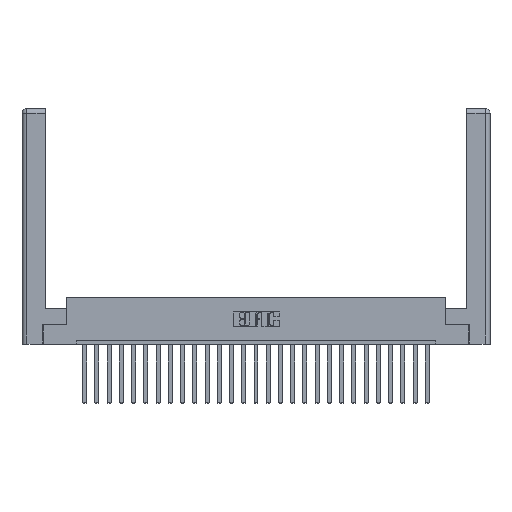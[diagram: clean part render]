
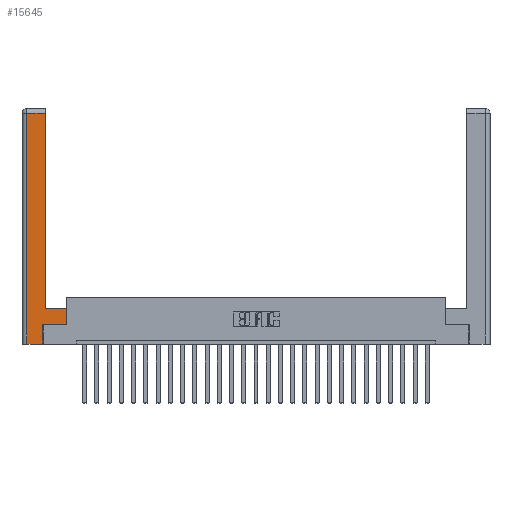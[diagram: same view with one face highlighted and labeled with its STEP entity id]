
A CAD part, top view. The second image highlights one B-rep face of the part: STEP entity #15645.
In plain terms, the highlighted planar face has unit normal (0, 0, 1).
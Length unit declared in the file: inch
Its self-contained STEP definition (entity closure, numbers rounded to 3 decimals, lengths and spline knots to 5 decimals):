
#399 = EDGE_CURVE ( 'NONE', #15824, #610, #18422, .T. ) ;
#425 = VERTEX_POINT ( 'NONE', #15621 ) ;
#495 = VECTOR ( 'NONE', #24600, 39.37008 ) ;
#610 = VERTEX_POINT ( 'NONE', #16352 ) ;
#700 = ORIENTED_EDGE ( 'NONE', *, *, #6892, .T. ) ;
#1013 = VECTOR ( 'NONE', #6196, 39.37008 ) ;
#1184 = VERTEX_POINT ( 'NONE', #17019 ) ;
#1859 = EDGE_CURVE ( 'NONE', #1184, #15824, #9740, .T. ) ;
#1968 = VERTEX_POINT ( 'NONE', #3947 ) ;
#2933 = ORIENTED_EDGE ( 'NONE', *, *, #16613, .T. ) ;
#3351 = ORIENTED_EDGE ( 'NONE', *, *, #1859, .T. ) ;
#3456 = CARTESIAN_POINT ( 'NONE',  ( 0., 0., 0. ) ) ;
#3850 = DIRECTION ( 'NONE',  ( 0., 1., 0. ) ) ;
#3947 = CARTESIAN_POINT ( 'NONE',  ( 0.295, 0.45, 0. ) ) ;
#5816 = LINE ( 'NONE', #20457, #495 ) ;
#6196 = DIRECTION ( 'NONE',  ( 0., -1., 0. ) ) ;
#6818 = DIRECTION ( 'NONE',  ( 1., 0., 0. ) ) ;
#6892 = EDGE_CURVE ( 'NONE', #16676, #21559, #5816, .T. ) ;
#8018 = DIRECTION ( 'NONE',  ( 1., 0., 0. ) ) ;
#8739 = VECTOR ( 'NONE', #8018, 39.37008 ) ;
#9120 = EDGE_CURVE ( 'NONE', #1968, #16676, #12401, .T. ) ;
#9267 = ORIENTED_EDGE ( 'NONE', *, *, #9120, .T. ) ;
#9740 = LINE ( 'NONE', #20321, #14400 ) ;
#9789 = VECTOR ( 'NONE', #11743, 39.37008 ) ;
#9829 = CARTESIAN_POINT ( 'NONE',  ( 0.565, 0.45, 0. ) ) ;
#10383 = EDGE_LOOP ( 'NONE', ( #9267, #700, #13866, #15862, #23009, #3351, #13496, #2933 ) ) ;
#10463 = VECTOR ( 'NONE', #19411, 39.37008 ) ;
#11362 = DIRECTION ( 'NONE',  ( -1., 0., 0. ) ) ;
#11571 = CARTESIAN_POINT ( 'NONE',  ( 0.265, 0., 0. ) ) ;
#11743 = DIRECTION ( 'NONE',  ( 0., 1., 0. ) ) ;
#11858 = CARTESIAN_POINT ( 'NONE',  ( 0.295, 2.94, 0. ) ) ;
#11982 = LINE ( 'NONE', #16423, #14141 ) ;
#12401 = LINE ( 'NONE', #25675, #13331 ) ;
#12723 = CARTESIAN_POINT ( 'NONE',  ( 0.0615, 0., 0. ) ) ;
#13331 = VECTOR ( 'NONE', #3850, 39.37008 ) ;
#13496 = ORIENTED_EDGE ( 'NONE', *, *, #399, .T. ) ;
#13695 = PLANE ( 'NONE',  #14970 ) ;
#13866 = ORIENTED_EDGE ( 'NONE', *, *, #17512, .T. ) ;
#14141 = VECTOR ( 'NONE', #14555, 39.37008 ) ;
#14400 = VECTOR ( 'NONE', #6818, 39.37008 ) ;
#14555 = DIRECTION ( 'NONE',  ( -1., 0., 0. ) ) ;
#14970 = AXIS2_PLACEMENT_3D ( 'NONE', #3456, #23194, #11362 ) ;
#15621 = CARTESIAN_POINT ( 'NONE',  ( 0.265, 0., 0. ) ) ;
#15645 = ADVANCED_FACE ( 'NONE', ( #22837 ), #13695, .F. ) ;
#15736 = VERTEX_POINT ( 'NONE', #12723 ) ;
#15824 = VERTEX_POINT ( 'NONE', #18900 ) ;
#15862 = ORIENTED_EDGE ( 'NONE', *, *, #19632, .T. ) ;
#16223 = CARTESIAN_POINT ( 'NONE',  ( 0.0615, 0., 0. ) ) ;
#16352 = CARTESIAN_POINT ( 'NONE',  ( 0.565, 0.45, 0. ) ) ;
#16423 = CARTESIAN_POINT ( 'NONE',  ( 0.295, 0.45, 0. ) ) ;
#16613 = EDGE_CURVE ( 'NONE', #610, #1968, #11982, .T. ) ;
#16676 = VERTEX_POINT ( 'NONE', #11858 ) ;
#17019 = CARTESIAN_POINT ( 'NONE',  ( 0.265, 0.245, 0. ) ) ;
#17512 = EDGE_CURVE ( 'NONE', #21559, #15736, #19309, .T. ) ;
#18422 = LINE ( 'NONE', #9829, #9789 ) ;
#18900 = CARTESIAN_POINT ( 'NONE',  ( 0.565, 0.245, 0. ) ) ;
#19309 = LINE ( 'NONE', #16223, #1013 ) ;
#19411 = DIRECTION ( 'NONE',  ( 0., 1., 0. ) ) ;
#19632 = EDGE_CURVE ( 'NONE', #15736, #425, #22632, .T. ) ;
#20321 = CARTESIAN_POINT ( 'NONE',  ( 0.565, 0.245, 0. ) ) ;
#20457 = CARTESIAN_POINT ( 'NONE',  ( 0.0615, 2.94, 0. ) ) ;
#21559 = VERTEX_POINT ( 'NONE', #23001 ) ;
#22632 = LINE ( 'NONE', #11571, #8739 ) ;
#22837 = FACE_OUTER_BOUND ( 'NONE', #10383, .T. ) ;
#23001 = CARTESIAN_POINT ( 'NONE',  ( 0.0615, 2.94, 0. ) ) ;
#23009 = ORIENTED_EDGE ( 'NONE', *, *, #25615, .T. ) ;
#23194 = DIRECTION ( 'NONE',  ( 0., 0., -1. ) ) ;
#23324 = CARTESIAN_POINT ( 'NONE',  ( 0.265, 0.245, 0. ) ) ;
#24600 = DIRECTION ( 'NONE',  ( -1., 0., 0. ) ) ;
#25615 = EDGE_CURVE ( 'NONE', #425, #1184, #25638, .T. ) ;
#25638 = LINE ( 'NONE', #23324, #10463 ) ;
#25675 = CARTESIAN_POINT ( 'NONE',  ( 0.295, 3., 0. ) ) ;
